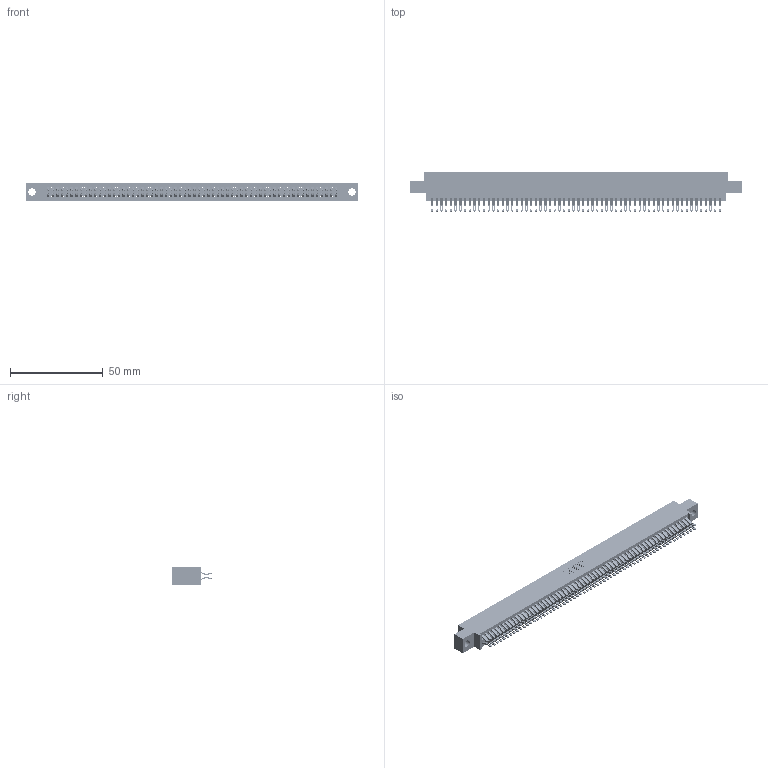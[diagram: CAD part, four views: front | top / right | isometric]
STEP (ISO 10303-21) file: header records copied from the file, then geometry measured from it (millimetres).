
FILE_DESCRIPTION (( 'STEP AP203' ), '1' );
FILE_NAME ('345-124-555-804.STEP', '2018-10-19T10:53:29', ( '' ), ( '' ), 'SwSTEP 2.0', 'SolidWorks 2016', '' );
FILE_SCHEMA (( 'CONFIG_CONTROL_DESIGN' ));
Length unit declared in the file: inch
Products named in the file (3): 345-292-001_555 Tail; 345 Part_0.170 Offset - 0.156 Dia-TH; 345-124-555-804
Assembly tree (125 placements, depth 2):
  345-124-555-804
    345 Part_0.170 Offset - 0.156 Dia-TH
    345-292-001_555 Tail  x124
Bounding box: 178.69 x 21.13 x 9.4 mm (x, y, z)
Volume: 17702.1 mm3; surface area: 27763.7 mm2
Topology: 125 solids, 125 shells, 7074 faces, 22301 edges, 14866 vertices
Faces by surface type: plane 3928, cylinder 3146
Entity records: 46415 total; most frequent: CARTESIAN_POINT 7798, ORIENTED_EDGE 7702, DIRECTION 6819, EDGE_CURVE 3851, LINE 3451, VECTOR 3451, VERTEX_POINT 2566, AXIS2_PLACEMENT_3D 1684
